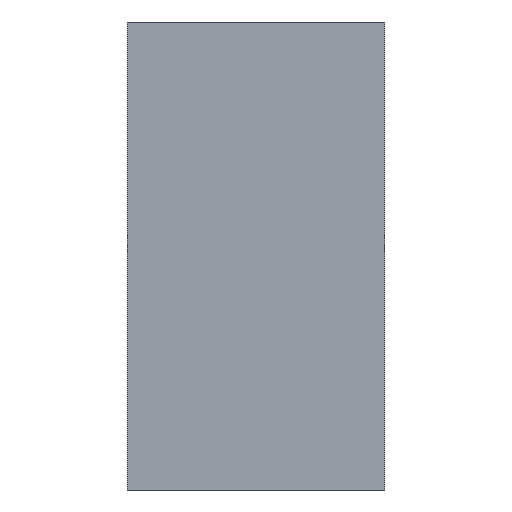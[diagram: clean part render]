
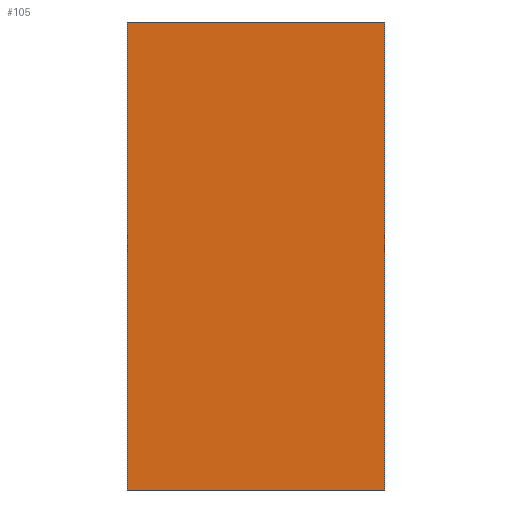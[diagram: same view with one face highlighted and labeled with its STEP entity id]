
A CAD part, front view. The second image highlights one B-rep face of the part: STEP entity #105.
In plain terms, the highlighted planar face has unit normal (0, -1, 0).
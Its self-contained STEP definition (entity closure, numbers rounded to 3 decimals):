
#11 = EDGE_LOOP ( 'NONE', ( #100, #99, #98, #97 ) ) ;
#17 = CARTESIAN_POINT ( 'NONE',  ( 5.5, 0., 0. ) ) ;
#18 = PLANE ( 'NONE',  #183 ) ;
#20 = CARTESIAN_POINT ( 'NONE',  ( 5.5, 0., 0. ) ) ;
#22 = CARTESIAN_POINT ( 'NONE',  ( 0., 0., -10. ) ) ;
#45 = VECTOR ( 'NONE', #277, 1000. ) ;
#47 = VECTOR ( 'NONE', #281, 1000. ) ;
#48 = LINE ( 'NONE', #278, #45 ) ;
#50 = LINE ( 'NONE', #283, #47 ) ;
#51 = VECTOR ( 'NONE', #286, 1000. ) ;
#54 = LINE ( 'NONE', #289, #51 ) ;
#63 = VECTOR ( 'NONE', #235, 1000. ) ;
#66 = LINE ( 'NONE', #239, #63 ) ;
#80 = FACE_OUTER_BOUND ( 'NONE', #11, .T. ) ;
#97 = ORIENTED_EDGE ( 'NONE', *, *, #198, .T. ) ;
#98 = ORIENTED_EDGE ( 'NONE', *, *, #201, .F. ) ;
#99 = ORIENTED_EDGE ( 'NONE', *, *, #192, .F. ) ;
#100 = ORIENTED_EDGE ( 'NONE', *, *, #200, .T. ) ;
#105 = ADVANCED_FACE ( 'NONE', ( #80 ), #18, .F. ) ;
#115 = VERTEX_POINT ( 'NONE', #294 ) ;
#116 = VERTEX_POINT ( 'NONE', #17 ) ;
#117 = VERTEX_POINT ( 'NONE', #22 ) ;
#120 = VERTEX_POINT ( 'NONE', #293 ) ;
#183 = AXIS2_PLACEMENT_3D ( 'NONE', #20, #231, #232 ) ;
#192 = EDGE_CURVE ( 'NONE', #120, #117, #66, .T. ) ;
#198 = EDGE_CURVE ( 'NONE', #116, #115, #54, .T. ) ;
#200 = EDGE_CURVE ( 'NONE', #115, #117, #50, .T. ) ;
#201 = EDGE_CURVE ( 'NONE', #116, #120, #48, .T. ) ;
#231 = DIRECTION ( 'NONE',  ( 0., 1., 0. ) ) ;
#232 = DIRECTION ( 'NONE',  ( 0., 0., 1. ) ) ;
#235 = DIRECTION ( 'NONE',  ( -1., 0., 0. ) ) ;
#239 = CARTESIAN_POINT ( 'NONE',  ( 5.5, 0., -10. ) ) ;
#277 = DIRECTION ( 'NONE',  ( 0., 0., -1. ) ) ;
#278 = CARTESIAN_POINT ( 'NONE',  ( 5.5, 0., 0. ) ) ;
#281 = DIRECTION ( 'NONE',  ( 0., 0., -1. ) ) ;
#283 = CARTESIAN_POINT ( 'NONE',  ( 0., 0., 0. ) ) ;
#286 = DIRECTION ( 'NONE',  ( -1., 0., 0. ) ) ;
#289 = CARTESIAN_POINT ( 'NONE',  ( 5.5, 0., 0. ) ) ;
#293 = CARTESIAN_POINT ( 'NONE',  ( 5.5, 0., -10. ) ) ;
#294 = CARTESIAN_POINT ( 'NONE',  ( 0., 0., 0. ) ) ;
